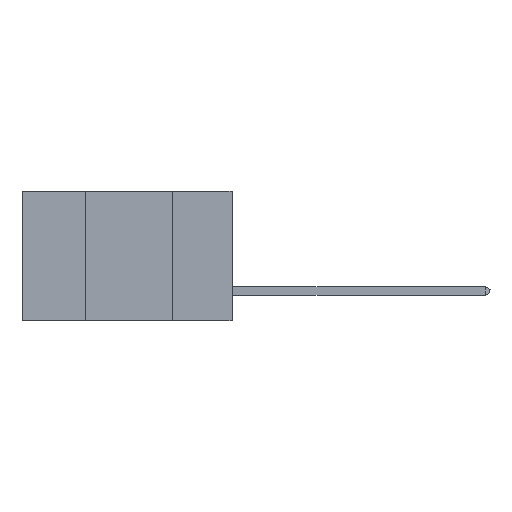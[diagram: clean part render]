
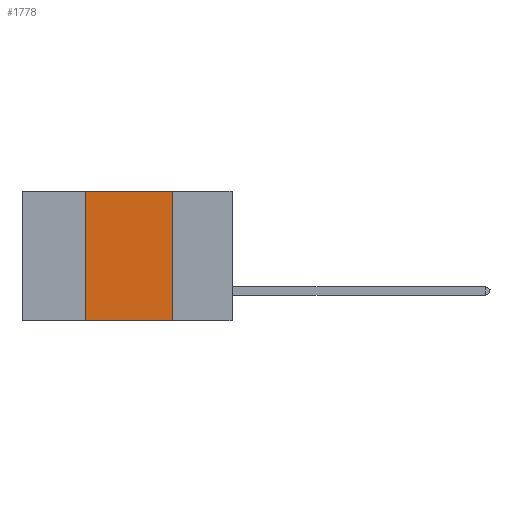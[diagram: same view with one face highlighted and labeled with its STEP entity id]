
A CAD part, left-side view. The second image highlights one B-rep face of the part: STEP entity #1778.
In plain terms, the highlighted planar face has unit normal (-1, 0, 0).
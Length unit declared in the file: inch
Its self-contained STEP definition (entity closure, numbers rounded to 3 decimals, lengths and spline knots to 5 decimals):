
#84 = AXIS2_PLACEMENT_3D ( 'NONE', #15262, #3828, #2933 ) ;
#305 = EDGE_CURVE ( 'NONE', #11430, #12213, #13893, .T. ) ;
#415 = CARTESIAN_POINT ( 'NONE',  ( 0., 0.17, 0. ) ) ;
#636 = DIRECTION ( 'NONE',  ( 0., 0., 1. ) ) ;
#1778 = ADVANCED_FACE ( 'NONE', ( #11778 ), #5106, .F. ) ;
#2519 = EDGE_CURVE ( 'NONE', #11430, #14169, #4930, .T. ) ;
#2933 = DIRECTION ( 'NONE',  ( 0., 0., -1. ) ) ;
#2942 = CARTESIAN_POINT ( 'NONE',  ( 0., 0.42, -0.37 ) ) ;
#3233 = EDGE_CURVE ( 'NONE', #12213, #14635, #7411, .T. ) ;
#3828 = DIRECTION ( 'NONE',  ( 1., 0., 0. ) ) ;
#4435 = VECTOR ( 'NONE', #9954, 39.37008 ) ;
#4930 = LINE ( 'NONE', #16699, #18302 ) ;
#5106 = PLANE ( 'NONE',  #84 ) ;
#5127 = ORIENTED_EDGE ( 'NONE', *, *, #3233, .F. ) ;
#5623 = DIRECTION ( 'NONE',  ( 0., 0., -1. ) ) ;
#5694 = VECTOR ( 'NONE', #636, 39.37008 ) ;
#6688 = ORIENTED_EDGE ( 'NONE', *, *, #2519, .T. ) ;
#7105 = VECTOR ( 'NONE', #5623, 39.37008 ) ;
#7174 = ORIENTED_EDGE ( 'NONE', *, *, #305, .F. ) ;
#7411 = LINE ( 'NONE', #18274, #4435 ) ;
#8507 = CARTESIAN_POINT ( 'NONE',  ( 0., 0.17, 0. ) ) ;
#9954 = DIRECTION ( 'NONE',  ( 0., -1., 0. ) ) ;
#10719 = EDGE_CURVE ( 'NONE', #14635, #14169, #15948, .T. ) ;
#10942 = DIRECTION ( 'NONE',  ( 0., -1., 0. ) ) ;
#11430 = VERTEX_POINT ( 'NONE', #2942 ) ;
#11778 = FACE_OUTER_BOUND ( 'NONE', #16852, .T. ) ;
#12213 = VERTEX_POINT ( 'NONE', #16048 ) ;
#13893 = LINE ( 'NONE', #15306, #5694 ) ;
#13901 = ORIENTED_EDGE ( 'NONE', *, *, #10719, .F. ) ;
#13958 = CARTESIAN_POINT ( 'NONE',  ( 0., 0.17, -0.37 ) ) ;
#14169 = VERTEX_POINT ( 'NONE', #13958 ) ;
#14635 = VERTEX_POINT ( 'NONE', #415 ) ;
#15262 = CARTESIAN_POINT ( 'NONE',  ( 0., 0.6, 0. ) ) ;
#15306 = CARTESIAN_POINT ( 'NONE',  ( 0., 0.42, 0. ) ) ;
#15948 = LINE ( 'NONE', #8507, #7105 ) ;
#16048 = CARTESIAN_POINT ( 'NONE',  ( 0., 0.42, 0. ) ) ;
#16699 = CARTESIAN_POINT ( 'NONE',  ( 0., 0.6, -0.37 ) ) ;
#16852 = EDGE_LOOP ( 'NONE', ( #13901, #5127, #7174, #6688 ) ) ;
#18274 = CARTESIAN_POINT ( 'NONE',  ( 0., 0.6, 0. ) ) ;
#18302 = VECTOR ( 'NONE', #10942, 39.37008 ) ;
